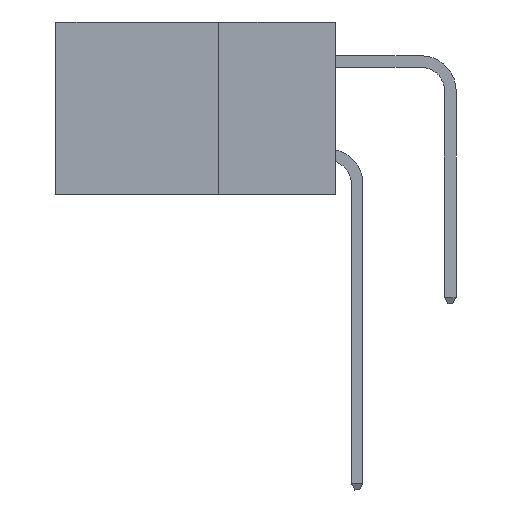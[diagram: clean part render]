
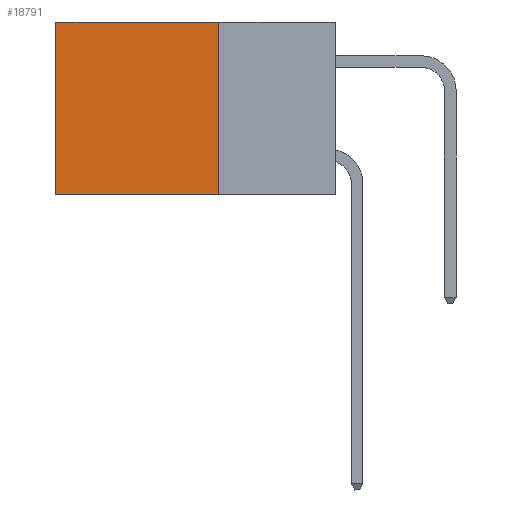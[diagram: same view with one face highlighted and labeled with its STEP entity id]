
A CAD part, left-side view. The second image highlights one B-rep face of the part: STEP entity #18791.
In plain terms, the highlighted planar face has unit normal (-1, 0, 0).
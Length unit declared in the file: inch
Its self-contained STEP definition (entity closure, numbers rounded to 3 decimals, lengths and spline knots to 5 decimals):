
#194 = LINE ( 'NONE', #1515, #20416 ) ;
#450 = FACE_OUTER_BOUND ( 'NONE', #16157, .T. ) ;
#982 = CARTESIAN_POINT ( 'NONE',  ( 0.2875, 0.6, -0.37 ) ) ;
#1515 = CARTESIAN_POINT ( 'NONE',  ( 0.2875, 0.6, 0. ) ) ;
#1717 = PLANE ( 'NONE',  #4482 ) ;
#1804 = ORIENTED_EDGE ( 'NONE', *, *, #3388, .F. ) ;
#2290 = VERTEX_POINT ( 'NONE', #16562 ) ;
#2553 = ORIENTED_EDGE ( 'NONE', *, *, #16074, .F. ) ;
#2878 = DIRECTION ( 'NONE',  ( 0., 0., -1. ) ) ;
#2952 = EDGE_CURVE ( 'NONE', #20593, #8586, #194, .T. ) ;
#3388 = EDGE_CURVE ( 'NONE', #22316, #2290, #9720, .T. ) ;
#4482 = AXIS2_PLACEMENT_3D ( 'NONE', #5598, #18730, #7464 ) ;
#4562 = CARTESIAN_POINT ( 'NONE',  ( 0.2875, 0.6, 0. ) ) ;
#5598 = CARTESIAN_POINT ( 'NONE',  ( 0.2875, 0.25, 0. ) ) ;
#5706 = VECTOR ( 'NONE', #10830, 39.37008 ) ;
#6311 = LINE ( 'NONE', #24081, #5706 ) ;
#7464 = DIRECTION ( 'NONE',  ( 0., 0., -1. ) ) ;
#7635 = ORIENTED_EDGE ( 'NONE', *, *, #2952, .T. ) ;
#7998 = EDGE_CURVE ( 'NONE', #22316, #20593, #6311, .T. ) ;
#8586 = VERTEX_POINT ( 'NONE', #982 ) ;
#9077 = DIRECTION ( 'NONE',  ( 0., 0., -1. ) ) ;
#9720 = LINE ( 'NONE', #10379, #19165 ) ;
#10379 = CARTESIAN_POINT ( 'NONE',  ( 0.2875, 0.25, 0. ) ) ;
#10830 = DIRECTION ( 'NONE',  ( 0., 1., 0. ) ) ;
#11796 = CARTESIAN_POINT ( 'NONE',  ( 0.2875, 0.25, 0. ) ) ;
#16040 = CARTESIAN_POINT ( 'NONE',  ( 0.2875, 0.25, -0.37 ) ) ;
#16074 = EDGE_CURVE ( 'NONE', #2290, #8586, #21677, .T. ) ;
#16157 = EDGE_LOOP ( 'NONE', ( #7635, #2553, #1804, #24314 ) ) ;
#16554 = VECTOR ( 'NONE', #17922, 39.37008 ) ;
#16562 = CARTESIAN_POINT ( 'NONE',  ( 0.2875, 0.25, -0.37 ) ) ;
#17922 = DIRECTION ( 'NONE',  ( 0., 1., 0. ) ) ;
#18730 = DIRECTION ( 'NONE',  ( 1., 0., 0. ) ) ;
#18791 = ADVANCED_FACE ( 'NONE', ( #450 ), #1717, .F. ) ;
#19165 = VECTOR ( 'NONE', #2878, 39.37008 ) ;
#20416 = VECTOR ( 'NONE', #9077, 39.37008 ) ;
#20593 = VERTEX_POINT ( 'NONE', #4562 ) ;
#21677 = LINE ( 'NONE', #16040, #16554 ) ;
#22316 = VERTEX_POINT ( 'NONE', #11796 ) ;
#24081 = CARTESIAN_POINT ( 'NONE',  ( 0.2875, 0.25, 0. ) ) ;
#24314 = ORIENTED_EDGE ( 'NONE', *, *, #7998, .T. ) ;
